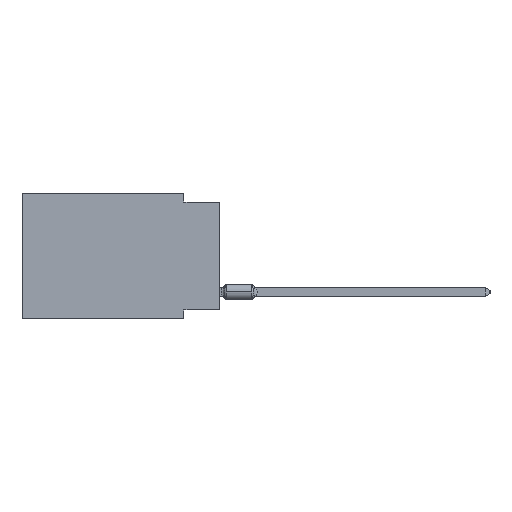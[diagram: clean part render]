
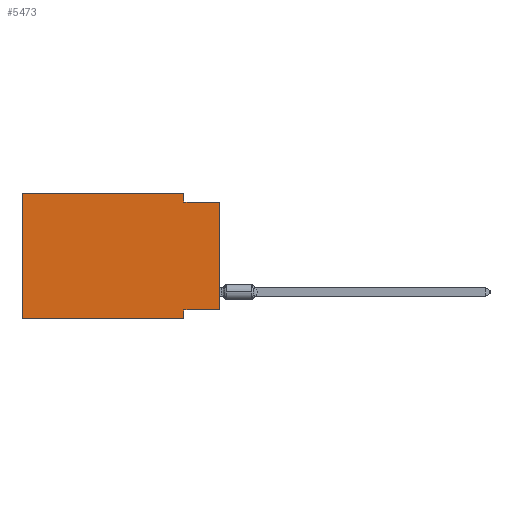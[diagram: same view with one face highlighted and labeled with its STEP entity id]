
A CAD part, left-side view. The second image highlights one B-rep face of the part: STEP entity #5473.
In plain terms, the highlighted planar face has unit normal (-1, 0, 0).
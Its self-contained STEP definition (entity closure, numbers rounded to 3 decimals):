
#209 = VECTOR ( 'NONE', #52066, 1000. ) ;
#1834 = CARTESIAN_POINT ( 'NONE',  ( 0., 2.54, -0.635 ) ) ;
#2303 = EDGE_CURVE ( 'NONE', #18527, #35014, #14891, .T. ) ;
#3049 = DIRECTION ( 'NONE',  ( 0., 1., 0. ) ) ;
#3843 = LINE ( 'NONE', #14782, #43257 ) ;
#5084 = LINE ( 'NONE', #66507, #70662 ) ;
#5473 = ADVANCED_FACE ( 'NONE', ( #50869 ), #50521, .F. ) ;
#5920 = ORIENTED_EDGE ( 'NONE', *, *, #61016, .F. ) ;
#6486 = LINE ( 'NONE', #61719, #28064 ) ;
#7371 = LINE ( 'NONE', #40271, #51367 ) ;
#12112 = ORIENTED_EDGE ( 'NONE', *, *, #48447, .F. ) ;
#14365 = CARTESIAN_POINT ( 'NONE',  ( 0., 0., -8.255 ) ) ;
#14782 = CARTESIAN_POINT ( 'NONE',  ( 0., 2.54, 0. ) ) ;
#14891 = LINE ( 'NONE', #26242, #60763 ) ;
#16334 = VERTEX_POINT ( 'NONE', #62742 ) ;
#17809 = DIRECTION ( 'NONE',  ( 0., 0., 1. ) ) ;
#18115 = VECTOR ( 'NONE', #3049, 1000. ) ;
#18527 = VERTEX_POINT ( 'NONE', #48614 ) ;
#19137 = LINE ( 'NONE', #14365, #18115 ) ;
#19842 = CARTESIAN_POINT ( 'NONE',  ( 0., 2.54, -8.89 ) ) ;
#22101 = CARTESIAN_POINT ( 'NONE',  ( 0., 13.97, -8.89 ) ) ;
#22768 = ORIENTED_EDGE ( 'NONE', *, *, #33935, .T. ) ;
#24002 = VECTOR ( 'NONE', #17809, 1000. ) ;
#25536 = CARTESIAN_POINT ( 'NONE',  ( 0., 2.54, -8.89 ) ) ;
#26242 = CARTESIAN_POINT ( 'NONE',  ( 0., 0., 0. ) ) ;
#26603 = DIRECTION ( 'NONE',  ( 0., 0., 1. ) ) ;
#28064 = VECTOR ( 'NONE', #28782, 1000. ) ;
#28541 = DIRECTION ( 'NONE',  ( 1., 0., 0. ) ) ;
#28782 = DIRECTION ( 'NONE',  ( 0., -1., 0. ) ) ;
#30210 = CARTESIAN_POINT ( 'NONE',  ( 0., 13.97, 0. ) ) ;
#33672 = CARTESIAN_POINT ( 'NONE',  ( 0., 13.97, 0. ) ) ;
#33935 = EDGE_CURVE ( 'NONE', #56938, #53053, #7371, .T. ) ;
#34377 = DIRECTION ( 'NONE',  ( 0., 0., -1. ) ) ;
#35014 = VERTEX_POINT ( 'NONE', #62305 ) ;
#35249 = CARTESIAN_POINT ( 'NONE',  ( 0., 2.54, 0. ) ) ;
#37094 = DIRECTION ( 'NONE',  ( 0., 0., -1. ) ) ;
#38396 = EDGE_LOOP ( 'NONE', ( #53927, #12112, #63601, #5920, #52358, #22768, #43179, #38676 ) ) ;
#38676 = ORIENTED_EDGE ( 'NONE', *, *, #53825, .F. ) ;
#40271 = CARTESIAN_POINT ( 'NONE',  ( 0., 13.97, -8.89 ) ) ;
#41359 = DIRECTION ( 'NONE',  ( 0., -1., 0. ) ) ;
#42525 = VERTEX_POINT ( 'NONE', #1834 ) ;
#43179 = ORIENTED_EDGE ( 'NONE', *, *, #66946, .F. ) ;
#43257 = VECTOR ( 'NONE', #37094, 1000. ) ;
#46311 = LINE ( 'NONE', #30210, #24002 ) ;
#48447 = EDGE_CURVE ( 'NONE', #42525, #35014, #5084, .T. ) ;
#48614 = CARTESIAN_POINT ( 'NONE',  ( 0., 0., -8.255 ) ) ;
#50055 = DIRECTION ( 'NONE',  ( 0., -1., 0. ) ) ;
#50521 = PLANE ( 'NONE',  #68120 ) ;
#50869 = FACE_OUTER_BOUND ( 'NONE', #38396, .T. ) ;
#51367 = VECTOR ( 'NONE', #41359, 1000. ) ;
#52066 = DIRECTION ( 'NONE',  ( 0., 0., -1. ) ) ;
#52358 = ORIENTED_EDGE ( 'NONE', *, *, #54564, .F. ) ;
#53053 = VERTEX_POINT ( 'NONE', #25536 ) ;
#53825 = EDGE_CURVE ( 'NONE', #18527, #63856, #19137, .T. ) ;
#53927 = ORIENTED_EDGE ( 'NONE', *, *, #2303, .T. ) ;
#54564 = EDGE_CURVE ( 'NONE', #56938, #16334, #46311, .T. ) ;
#54997 = VERTEX_POINT ( 'NONE', #35249 ) ;
#56938 = VERTEX_POINT ( 'NONE', #22101 ) ;
#60763 = VECTOR ( 'NONE', #26603, 1000. ) ;
#61016 = EDGE_CURVE ( 'NONE', #16334, #54997, #6486, .T. ) ;
#61719 = CARTESIAN_POINT ( 'NONE',  ( 0., 13.97, 0. ) ) ;
#62305 = CARTESIAN_POINT ( 'NONE',  ( 0., 0., -0.635 ) ) ;
#62742 = CARTESIAN_POINT ( 'NONE',  ( 0., 13.97, 0. ) ) ;
#63031 = LINE ( 'NONE', #19842, #209 ) ;
#63601 = ORIENTED_EDGE ( 'NONE', *, *, #65464, .F. ) ;
#63856 = VERTEX_POINT ( 'NONE', #72380 ) ;
#65464 = EDGE_CURVE ( 'NONE', #54997, #42525, #3843, .T. ) ;
#66507 = CARTESIAN_POINT ( 'NONE',  ( 0., 0., -0.635 ) ) ;
#66946 = EDGE_CURVE ( 'NONE', #63856, #53053, #63031, .T. ) ;
#68120 = AXIS2_PLACEMENT_3D ( 'NONE', #33672, #28541, #34377 ) ;
#70662 = VECTOR ( 'NONE', #50055, 1000. ) ;
#72380 = CARTESIAN_POINT ( 'NONE',  ( 0., 2.54, -8.255 ) ) ;
